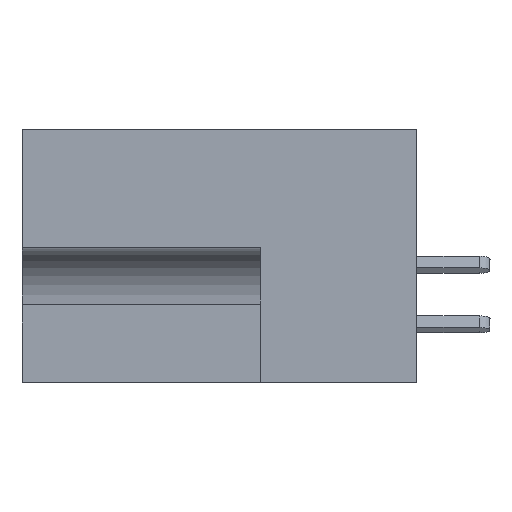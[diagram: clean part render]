
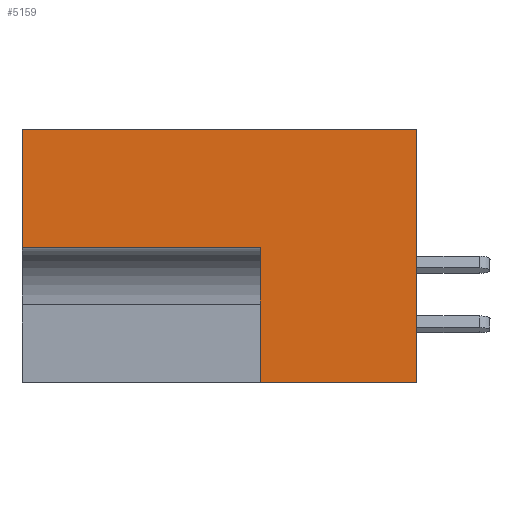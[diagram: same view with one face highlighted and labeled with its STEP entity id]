
A CAD part, left-side view. The second image highlights one B-rep face of the part: STEP entity #5159.
In plain terms, the highlighted planar face has unit normal (-1, 0, 0).
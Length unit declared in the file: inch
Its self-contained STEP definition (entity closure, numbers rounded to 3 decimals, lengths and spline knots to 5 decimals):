
#195 = CARTESIAN_POINT ( 'NONE',  ( 0., 0.328, -0.531 ) ) ;
#986 = EDGE_CURVE ( 'NONE', #10286, #2938, #4822, .T. ) ;
#1033 = ORIENTED_EDGE ( 'NONE', *, *, #3160, .F. ) ;
#1099 = DIRECTION ( 'NONE',  ( 0., 0., 1. ) ) ;
#1394 = CARTESIAN_POINT ( 'NONE',  ( 0., 0.828, 0. ) ) ;
#1785 = CARTESIAN_POINT ( 'NONE',  ( 0., 0.328, -0.248 ) ) ;
#2560 = ORIENTED_EDGE ( 'NONE', *, *, #9227, .F. ) ;
#2564 = DIRECTION ( 'NONE',  ( 0., 0., -1. ) ) ;
#2861 = VECTOR ( 'NONE', #1099, 39.37008 ) ;
#2922 = CARTESIAN_POINT ( 'NONE',  ( 0., 0., 0. ) ) ;
#2938 = VERTEX_POINT ( 'NONE', #11628 ) ;
#3160 = EDGE_CURVE ( 'NONE', #6414, #23249, #15762, .T. ) ;
#3294 = DIRECTION ( 'NONE',  ( 0., 1., 0. ) ) ;
#3304 = ORIENTED_EDGE ( 'NONE', *, *, #3966, .T. ) ;
#3913 = EDGE_CURVE ( 'NONE', #10027, #2938, #19156, .T. ) ;
#3966 = EDGE_CURVE ( 'NONE', #7372, #10286, #17170, .T. ) ;
#4124 = DIRECTION ( 'NONE',  ( 0., -1., 0. ) ) ;
#4511 = CARTESIAN_POINT ( 'NONE',  ( 0., 0.328, -0.531 ) ) ;
#4621 = LINE ( 'NONE', #16025, #6896 ) ;
#4822 = LINE ( 'NONE', #2922, #2861 ) ;
#5159 = ADVANCED_FACE ( 'NONE', ( #18150 ), #22457, .F. ) ;
#6414 = VERTEX_POINT ( 'NONE', #6474 ) ;
#6474 = CARTESIAN_POINT ( 'NONE',  ( 0., 0.328, -0.248 ) ) ;
#6690 = CARTESIAN_POINT ( 'NONE',  ( 0., 0.453, 0. ) ) ;
#6896 = VECTOR ( 'NONE', #19694, 39.37008 ) ;
#7372 = VERTEX_POINT ( 'NONE', #195 ) ;
#7500 = CARTESIAN_POINT ( 'NONE',  ( 0., 0., -0.531 ) ) ;
#9227 = EDGE_CURVE ( 'NONE', #7372, #6414, #12001, .T. ) ;
#9763 = CARTESIAN_POINT ( 'NONE',  ( 0., 0.828, -0.248 ) ) ;
#10027 = VERTEX_POINT ( 'NONE', #1394 ) ;
#10262 = DIRECTION ( 'NONE',  ( 1., 0., 0. ) ) ;
#10286 = VERTEX_POINT ( 'NONE', #7500 ) ;
#11628 = CARTESIAN_POINT ( 'NONE',  ( 0., 0., 0. ) ) ;
#12001 = LINE ( 'NONE', #4511, #16808 ) ;
#12620 = EDGE_CURVE ( 'NONE', #23249, #10027, #4621, .T. ) ;
#13720 = ORIENTED_EDGE ( 'NONE', *, *, #3913, .F. ) ;
#14263 = EDGE_LOOP ( 'NONE', ( #17587, #1033, #2560, #3304, #20186, #13720 ) ) ;
#15210 = DIRECTION ( 'NONE',  ( 0., 0., 1. ) ) ;
#15762 = LINE ( 'NONE', #1785, #16915 ) ;
#16025 = CARTESIAN_POINT ( 'NONE',  ( 0., 0.828, 0. ) ) ;
#16706 = CARTESIAN_POINT ( 'NONE',  ( 0., 0.453, -0.531 ) ) ;
#16808 = VECTOR ( 'NONE', #15210, 39.37008 ) ;
#16915 = VECTOR ( 'NONE', #3294, 39.37008 ) ;
#17170 = LINE ( 'NONE', #16706, #23400 ) ;
#17587 = ORIENTED_EDGE ( 'NONE', *, *, #12620, .F. ) ;
#17725 = AXIS2_PLACEMENT_3D ( 'NONE', #6690, #10262, #2564 ) ;
#18150 = FACE_OUTER_BOUND ( 'NONE', #14263, .T. ) ;
#18526 = DIRECTION ( 'NONE',  ( 0., -1., 0. ) ) ;
#19156 = LINE ( 'NONE', #22016, #19449 ) ;
#19449 = VECTOR ( 'NONE', #4124, 39.37008 ) ;
#19694 = DIRECTION ( 'NONE',  ( 0., 0., 1. ) ) ;
#20186 = ORIENTED_EDGE ( 'NONE', *, *, #986, .T. ) ;
#22016 = CARTESIAN_POINT ( 'NONE',  ( 0., 0.453, 0. ) ) ;
#22457 = PLANE ( 'NONE',  #17725 ) ;
#23249 = VERTEX_POINT ( 'NONE', #9763 ) ;
#23400 = VECTOR ( 'NONE', #18526, 39.37008 ) ;
